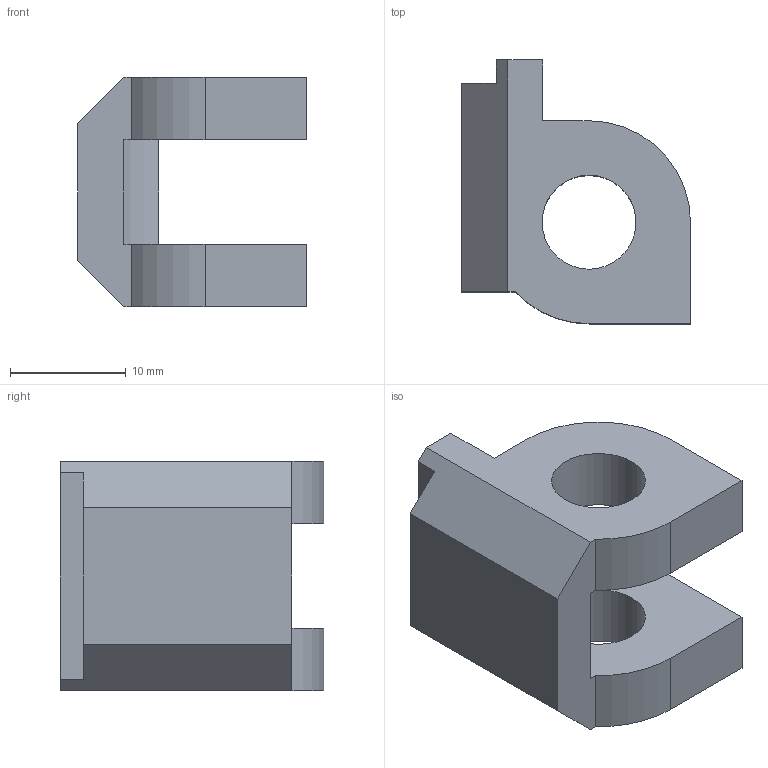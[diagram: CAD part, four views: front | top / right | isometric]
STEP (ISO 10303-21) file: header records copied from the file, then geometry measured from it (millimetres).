
FILE_DESCRIPTION((''),'2;1');
FILE_NAME('PM422FiringPinRetainer2.stp','2015-08-22T19:06:51',('JamesRPatrick'),(''),'Autodesk Inventor 2012','Autodesk Inventor 2012','');
FILE_SCHEMA(('AUTOMOTIVE_DESIGN { 1 0 10303 214 1 1 1 1 }'));
Length unit declared in the file: millimetre
Products named in the file (1): PM422FiringPinRetainer2
Bounding box: 19.75 x 22.75 x 19.8 mm (x, y, z)
Volume: 3595 mm3; surface area: 2485.2 mm2
Topology: 1 solids, 1 shells, 26 faces, 72 edges, 48 vertices
Faces by surface type: plane 19, cylinder 7
Full cylindrical faces by diameter (mm): 8.1 x2
Entity records: 854 total; most frequent: CARTESIAN_POINT 145, ORIENTED_EDGE 140, DIRECTION 138, EDGE_CURVE 70, VECTOR 56, LINE 56, VERTEX_POINT 48, AXIS2_PLACEMENT_3D 41
